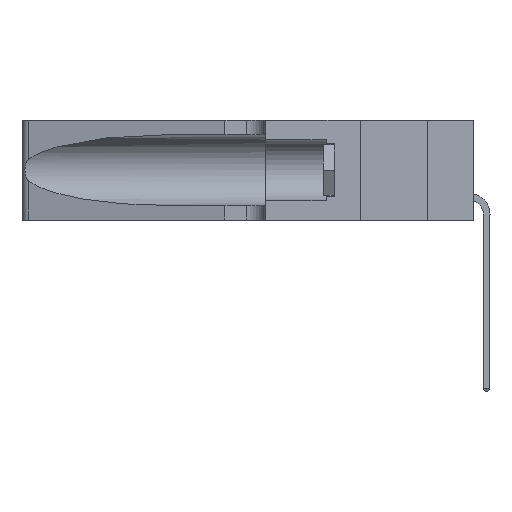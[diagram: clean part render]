
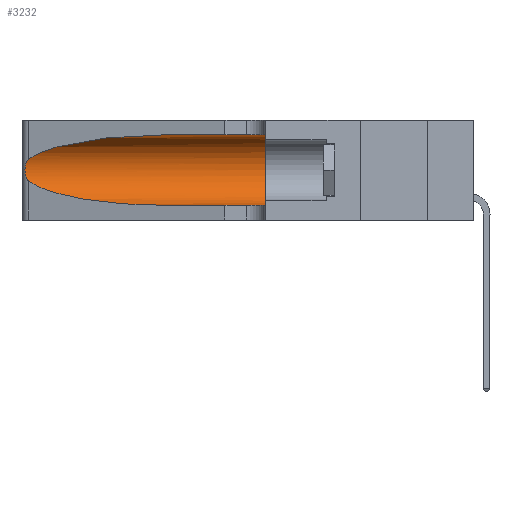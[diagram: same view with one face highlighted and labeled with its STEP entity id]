
A CAD part, left-side view. The second image highlights one B-rep face of the part: STEP entity #3232.
In plain terms, the highlighted cylindrical face has radius 3.308 mm (diameter 6.617 mm), a partial arc.
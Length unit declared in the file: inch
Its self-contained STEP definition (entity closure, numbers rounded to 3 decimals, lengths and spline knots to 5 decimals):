
#363 =( BOUNDED_CURVE ( )  B_SPLINE_CURVE ( 3, ( #6000, #1642, #3025, #15036 ),
 .UNSPECIFIED., .F., .T. ) 
 B_SPLINE_CURVE_WITH_KNOTS ( ( 4, 4 ),
 ( 3.44316, 4.71239 ),
 .UNSPECIFIED. ) 
 CURVE ( )  GEOMETRIC_REPRESENTATION_ITEM ( )  RATIONAL_B_SPLINE_CURVE ( ( 1., 0.87, 0.87, 1. ) ) 
 REPRESENTATION_ITEM ( '' )  );
#425 = CARTESIAN_POINT ( 'NONE',  ( 0.25789, 1.23486, 0.15765 ) ) ;
#1475 = CARTESIAN_POINT ( 'NONE',  ( 0.1305, 0.72297, 0.31525 ) ) ;
#1642 = CARTESIAN_POINT ( 'NONE',  ( 0.2373, 1.15595, 0.08982 ) ) ;
#1921 = DIRECTION ( 'NONE',  ( 0., 0., 1. ) ) ;
#1935 = CARTESIAN_POINT ( 'NONE',  ( 0.25639, 1.23186, 0.15144 ) ) ;
#2111 = EDGE_CURVE ( 'NONE', #16100, #7120, #16622, .T. ) ;
#2396 =( BOUNDED_CURVE ( )  B_SPLINE_CURVE ( 3, ( #1475, #19123, #7174, #10316 ),
 .UNSPECIFIED., .F., .F. ) 
 B_SPLINE_CURVE_WITH_KNOTS ( ( 4, 4 ),
 ( 1.5708, 2.84003 ),
 .UNSPECIFIED. ) 
 CURVE ( )  GEOMETRIC_REPRESENTATION_ITEM ( )  RATIONAL_B_SPLINE_CURVE ( ( 1., 0.87, 0.87, 1. ) ) 
 REPRESENTATION_ITEM ( '' )  );
#2522 = EDGE_CURVE ( 'NONE', #8885, #19019, #6329, .T. ) ;
#2624 = CARTESIAN_POINT ( 'NONE',  ( 0.1305, 0.72297, 0.31525 ) ) ;
#3025 = CARTESIAN_POINT ( 'NONE',  ( 0.18966, 0.96281, 0.05475 ) ) ;
#3232 = ADVANCED_FACE ( 'NONE', ( #11015 ), #4320, .F. ) ;
#3418 = CARTESIAN_POINT ( 'NONE',  ( 0.25639, 1.23184, 0.21858 ) ) ;
#3574 = DIRECTION ( 'NONE',  ( 0., -1., 0. ) ) ;
#4320 = CYLINDRICAL_SURFACE ( 'NONE', #10664, 0.13025 ) ;
#5165 = CARTESIAN_POINT ( 'NONE',  ( 0.26075, 1.23896, 0.178 ) ) ;
#5328 = VERTEX_POINT ( 'NONE', #11390 ) ;
#5910 = CARTESIAN_POINT ( 'NONE',  ( 0.1305, 0.35, 0.05475 ) ) ;
#6000 = CARTESIAN_POINT ( 'NONE',  ( 0.25487, 1.22718, 0.14631 ) ) ;
#6251 = ORIENTED_EDGE ( 'NONE', *, *, #10234, .F. ) ;
#6329 = B_SPLINE_CURVE_WITH_KNOTS ( 'NONE', 3,
 ( #13843, #12272, #3418, #16725, #10955, #18390, #11025, #5165, #16968, #18457, #425, #1935, #15241, #13780 ),
 .UNSPECIFIED., .F., .F.,
 ( 4, 2, 2, 2, 2, 2, 4 ),
 ( 0., 0.00027, 0.00053, 0.00107, 0.0016, 0.00187, 0.00214 ),
 .UNSPECIFIED. ) ;
#6384 = DIRECTION ( 'NONE',  ( 0., 1., 0. ) ) ;
#7120 = VERTEX_POINT ( 'NONE', #15924 ) ;
#7174 = CARTESIAN_POINT ( 'NONE',  ( 0.2373, 1.15595, 0.28018 ) ) ;
#7828 = LINE ( 'NONE', #10704, #17764 ) ;
#8219 = DIRECTION ( 'NONE',  ( 0., 0., -1. ) ) ;
#8298 = CARTESIAN_POINT ( 'NONE',  ( 0.1305, 1.61858, 0.185 ) ) ;
#8771 = VECTOR ( 'NONE', #19135, 39.37008 ) ;
#8885 = VERTEX_POINT ( 'NONE', #11962 ) ;
#9274 = CARTESIAN_POINT ( 'NONE',  ( 0.25487, 1.22718, 0.14631 ) ) ;
#9496 = ORIENTED_EDGE ( 'NONE', *, *, #12262, .T. ) ;
#9755 = VERTEX_POINT ( 'NONE', #5910 ) ;
#9978 = EDGE_CURVE ( 'NONE', #16100, #8885, #2396, .T. ) ;
#10061 = CIRCLE ( 'NONE', #18675, 0.13025 ) ;
#10234 = EDGE_CURVE ( 'NONE', #7120, #9755, #10061, .T. ) ;
#10316 = CARTESIAN_POINT ( 'NONE',  ( 0.25487, 1.22718, 0.22369 ) ) ;
#10664 = AXIS2_PLACEMENT_3D ( 'NONE', #8298, #17065, #8219 ) ;
#10704 = CARTESIAN_POINT ( 'NONE',  ( 0.1305, 1.61858, 0.05475 ) ) ;
#10955 = CARTESIAN_POINT ( 'NONE',  ( 0.25854, 1.2359, 0.20912 ) ) ;
#11015 = FACE_OUTER_BOUND ( 'NONE', #16535, .T. ) ;
#11025 = CARTESIAN_POINT ( 'NONE',  ( 0.26075, 1.23896, 0.19203 ) ) ;
#11390 = CARTESIAN_POINT ( 'NONE',  ( 0.1305, 0.72297, 0.05475 ) ) ;
#11962 = CARTESIAN_POINT ( 'NONE',  ( 0.25487, 1.22718, 0.22369 ) ) ;
#12086 = EDGE_CURVE ( 'NONE', #5328, #9755, #7828, .T. ) ;
#12262 = EDGE_CURVE ( 'NONE', #19019, #5328, #363, .T. ) ;
#12272 = CARTESIAN_POINT ( 'NONE',  ( 0.25555, 1.22994, 0.2215 ) ) ;
#13708 = CARTESIAN_POINT ( 'NONE',  ( 0.1305, 0.35, 0.185 ) ) ;
#13780 = CARTESIAN_POINT ( 'NONE',  ( 0.25487, 1.22718, 0.14631 ) ) ;
#13843 = CARTESIAN_POINT ( 'NONE',  ( 0.25487, 1.22718, 0.22369 ) ) ;
#14877 = CARTESIAN_POINT ( 'NONE',  ( 0.1305, 1.61858, 0.31525 ) ) ;
#15036 = CARTESIAN_POINT ( 'NONE',  ( 0.1305, 0.72297, 0.05475 ) ) ;
#15241 = CARTESIAN_POINT ( 'NONE',  ( 0.25555, 1.22993, 0.14849 ) ) ;
#15914 = ORIENTED_EDGE ( 'NONE', *, *, #12086, .T. ) ;
#15924 = CARTESIAN_POINT ( 'NONE',  ( 0.1305, 0.35, 0.31525 ) ) ;
#16100 = VERTEX_POINT ( 'NONE', #2624 ) ;
#16535 = EDGE_LOOP ( 'NONE', ( #18661, #17754, #9496, #15914, #6251, #18064 ) ) ;
#16622 = LINE ( 'NONE', #14877, #8771 ) ;
#16725 = CARTESIAN_POINT ( 'NONE',  ( 0.25787, 1.23484, 0.2124 ) ) ;
#16968 = CARTESIAN_POINT ( 'NONE',  ( 0.26017, 1.23833, 0.17102 ) ) ;
#17065 = DIRECTION ( 'NONE',  ( 0., -1., 0. ) ) ;
#17754 = ORIENTED_EDGE ( 'NONE', *, *, #2522, .T. ) ;
#17764 = VECTOR ( 'NONE', #3574, 39.37008 ) ;
#18064 = ORIENTED_EDGE ( 'NONE', *, *, #2111, .F. ) ;
#18390 = CARTESIAN_POINT ( 'NONE',  ( 0.26018, 1.23835, 0.19895 ) ) ;
#18457 = CARTESIAN_POINT ( 'NONE',  ( 0.25856, 1.23593, 0.16098 ) ) ;
#18661 = ORIENTED_EDGE ( 'NONE', *, *, #9978, .T. ) ;
#18675 = AXIS2_PLACEMENT_3D ( 'NONE', #13708, #6384, #1921 ) ;
#19019 = VERTEX_POINT ( 'NONE', #9274 ) ;
#19123 = CARTESIAN_POINT ( 'NONE',  ( 0.18966, 0.96281, 0.31525 ) ) ;
#19135 = DIRECTION ( 'NONE',  ( 0., -1., 0. ) ) ;
